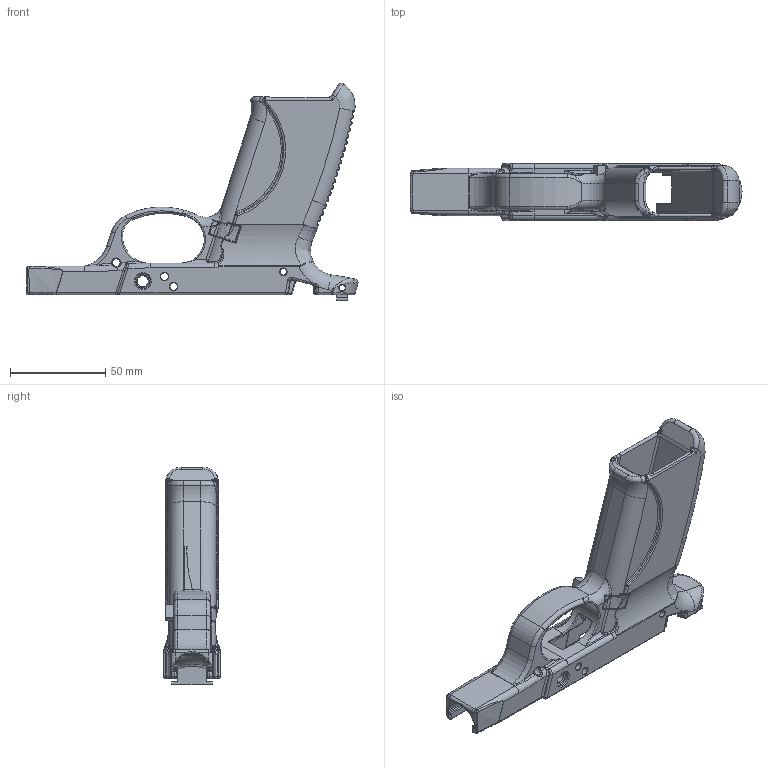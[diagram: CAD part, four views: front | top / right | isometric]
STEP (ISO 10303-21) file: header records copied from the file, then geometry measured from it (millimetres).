
FILE_DESCRIPTION(/* description */ (''),/* implementation_level */ '2;1');
FILE_NAME(/* name */ 'SR9CX.step',/* time_stamp */ '2019-11-17T18:03:33-05:00',/* author */ (''),/* organization */ (''),/* preprocessor_version */ 'ST-DEVELOPER v18',/* originating_system */ 'Autodesk Translation Framework v8.12.0.6',/* authorisation */ '');
FILE_SCHEMA (('AUTOMOTIVE_DESIGN { 1 0 10303 214 3 1 1 }'));
Products named in the file (3): SR9C; Mag Catch SR9; SR9 Rear Rail
Assembly tree (2 placements, depth 2):
  SR9C
    Mag Catch SR9
    SR9 Rear Rail
Bounding box: 174.67 x 30 x 114.42 mm (x, y, z)
Volume: 81767.4 mm3; surface area: 49486.3 mm2
Topology: 3 solids, 3 shells, 1497 faces, 3563 edges, 1975 vertices
Faces by surface type: cylinder 526, bspline 504, plane 200, torus 197, sphere 43, cone 27
Full cylindrical faces by diameter (mm): 3.175 x3, 3.5 x1, 4 x6, 4.36 x1, 5.8 x2, 8 x1
Entity records: 60744 total; most frequent: CARTESIAN_POINT 28670, ORIENTED_EDGE 6966, DIRECTION 6361, EDGE_CURVE 3483, AXIS2_PLACEMENT_3D 2636, VERTEX_POINT 1977, EDGE_LOOP 1518, FACE_OUTER_BOUND 1497
